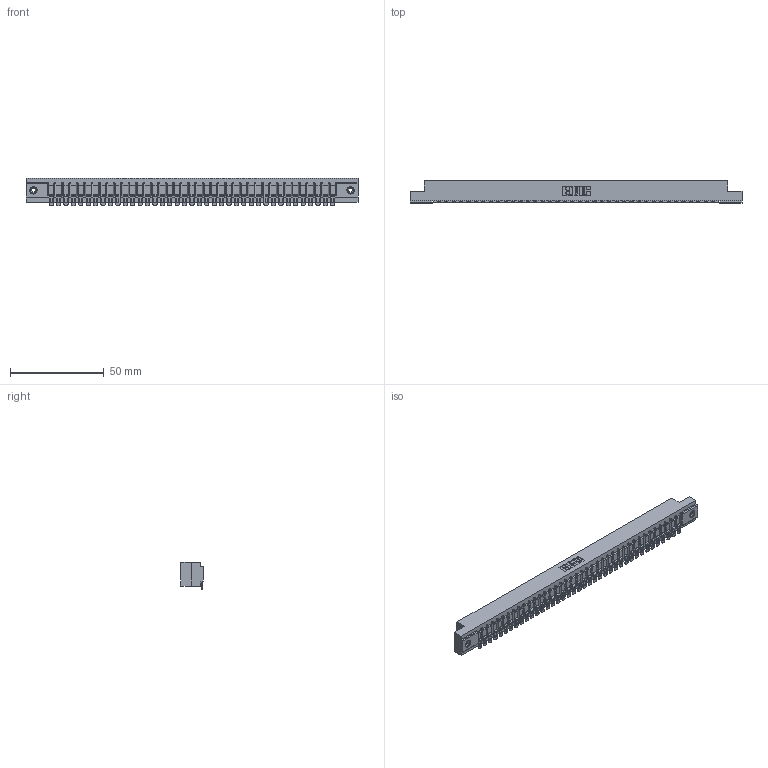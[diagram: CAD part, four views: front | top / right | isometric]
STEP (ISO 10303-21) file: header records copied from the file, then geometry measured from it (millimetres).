
FILE_DESCRIPTION (( 'STEP AP203' ), '1' );
FILE_NAME ('307-039-554-108.STEP', '2018-08-05T13:15:48', ( '' ), ( '' ), 'SwSTEP 2.0', 'SolidWorks 2016', '' );
FILE_SCHEMA (( 'CONFIG_CONTROL_DESIGN' ));
Length unit declared in the file: inch
Products named in the file (4): 307-039-554-108; 307 Part_.156 Dia Mounting Holes; 307-290-002_554; 345-250-001_345-250-003-102
Assembly tree (42 placements, depth 2):
  307-039-554-108
    307 Part_.156 Dia Mounting Holes
    307-290-002_554  x39
    345-250-001_345-250-003-102  x2
Bounding box: 177.55 x 12.01 x 14.52 mm (x, y, z)
Volume: 18984.8 mm3; surface area: 23974.8 mm2
Topology: 42 solids, 42 shells, 3377 faces, 10326 edges, 6768 vertices
Faces by surface type: plane 1896, cylinder 1385, sphere 80, cone 12, torus 4
Entity records: 35954 total; most frequent: CARTESIAN_POINT 6045, ORIENTED_EDGE 6028, DIRECTION 5890, EDGE_CURVE 3014, VECTOR 2300, LINE 2300, VERTEX_POINT 1950, AXIS2_PLACEMENT_3D 1795
